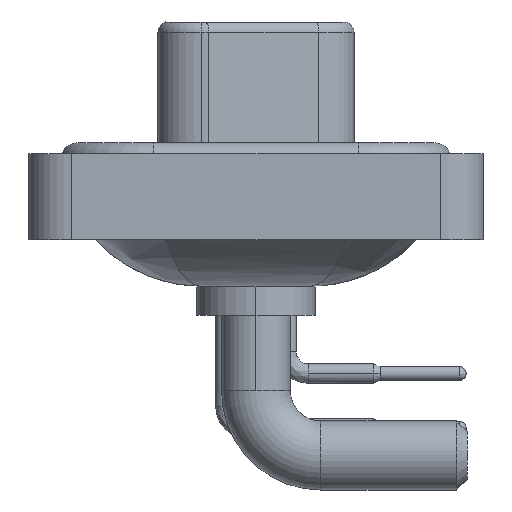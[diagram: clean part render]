
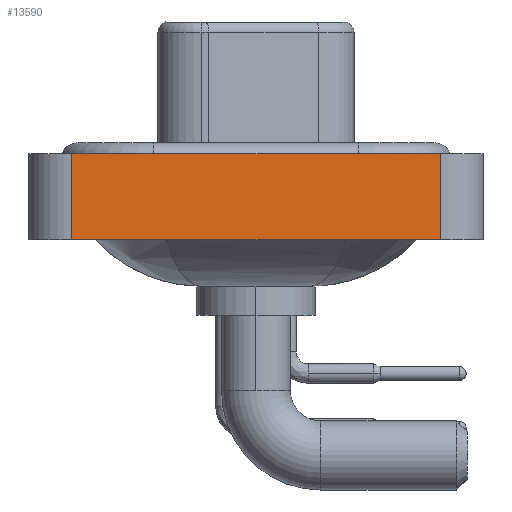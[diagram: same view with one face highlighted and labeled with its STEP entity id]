
A CAD part, left-side view. The second image highlights one B-rep face of the part: STEP entity #13590.
In plain terms, the highlighted planar face has unit normal (-1, 0, 0).
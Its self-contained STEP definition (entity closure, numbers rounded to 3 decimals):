
#683 = EDGE_CURVE ( 'NONE', #23916, #23515, #1266, .T. ) ;
#976 = ORIENTED_EDGE ( 'NONE', *, *, #683, .T. ) ;
#1266 = LINE ( 'NONE', #8598, #13390 ) ;
#1339 = ORIENTED_EDGE ( 'NONE', *, *, #15588, .F. ) ;
#5593 = ORIENTED_EDGE ( 'NONE', *, *, #9378, .T. ) ;
#5855 = CARTESIAN_POINT ( 'NONE',  ( -7.3, -8.55, -3.6 ) ) ;
#6614 = DIRECTION ( 'NONE',  ( 0., -1., 0. ) ) ;
#7016 = DIRECTION ( 'NONE',  ( 0., 0., 1. ) ) ;
#7233 = LINE ( 'NONE', #5855, #11505 ) ;
#8598 = CARTESIAN_POINT ( 'NONE',  ( -7.3, -8.55, -3.6 ) ) ;
#8880 = PLANE ( 'NONE',  #10932 ) ;
#9378 = EDGE_CURVE ( 'NONE', #23515, #10969, #7233, .T. ) ;
#9533 = VECTOR ( 'NONE', #17054, 1000. ) ;
#10932 = AXIS2_PLACEMENT_3D ( 'NONE', #14450, #16448, #7016 ) ;
#10969 = VERTEX_POINT ( 'NONE', #11166 ) ;
#11166 = CARTESIAN_POINT ( 'NONE',  ( -7.3, -8.55, 0.4 ) ) ;
#11460 = CARTESIAN_POINT ( 'NONE',  ( -7.3, -8.55, 0.4 ) ) ;
#11505 = VECTOR ( 'NONE', #18803, 1000. ) ;
#12852 = VECTOR ( 'NONE', #23152, 1000. ) ;
#13196 = LINE ( 'NONE', #11460, #9533 ) ;
#13390 = VECTOR ( 'NONE', #6614, 1000. ) ;
#13590 = ADVANCED_FACE ( 'NONE', ( #18458 ), #8880, .T. ) ;
#14450 = CARTESIAN_POINT ( 'NONE',  ( -7.3, -8.55, -3.6 ) ) ;
#14691 = CARTESIAN_POINT ( 'NONE',  ( -7.3, 8.55, 0.4 ) ) ;
#15588 = EDGE_CURVE ( 'NONE', #23916, #24394, #17185, .T. ) ;
#15920 = CARTESIAN_POINT ( 'NONE',  ( -7.3, -8.55, -3.6 ) ) ;
#15975 = ORIENTED_EDGE ( 'NONE', *, *, #17045, .F. ) ;
#16448 = DIRECTION ( 'NONE',  ( -1., 0., 0. ) ) ;
#17045 = EDGE_CURVE ( 'NONE', #24394, #10969, #13196, .T. ) ;
#17054 = DIRECTION ( 'NONE',  ( 0., -1., 0. ) ) ;
#17185 = LINE ( 'NONE', #20921, #12852 ) ;
#18458 = FACE_OUTER_BOUND ( 'NONE', #23086, .T. ) ;
#18803 = DIRECTION ( 'NONE',  ( 0., 0., 1. ) ) ;
#20921 = CARTESIAN_POINT ( 'NONE',  ( -7.3, 8.55, -3.6 ) ) ;
#23086 = EDGE_LOOP ( 'NONE', ( #5593, #15975, #1339, #976 ) ) ;
#23152 = DIRECTION ( 'NONE',  ( 0., 0., 1. ) ) ;
#23515 = VERTEX_POINT ( 'NONE', #15920 ) ;
#23621 = CARTESIAN_POINT ( 'NONE',  ( -7.3, 8.55, -3.6 ) ) ;
#23916 = VERTEX_POINT ( 'NONE', #23621 ) ;
#24394 = VERTEX_POINT ( 'NONE', #14691 ) ;
